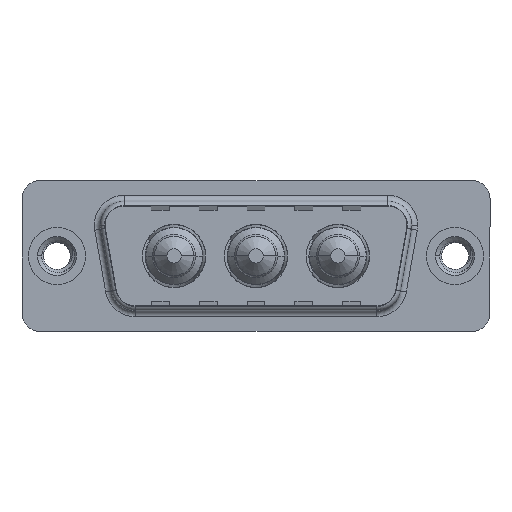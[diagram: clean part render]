
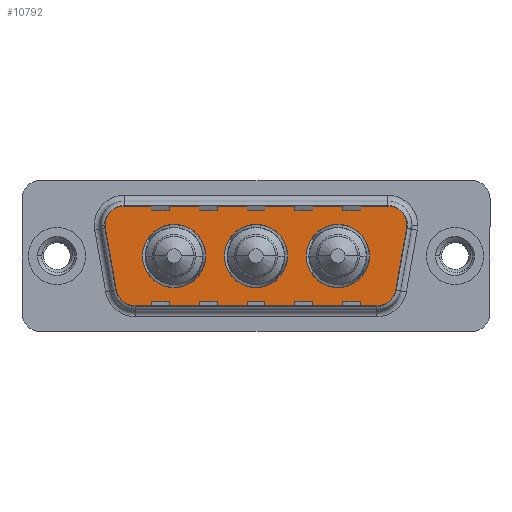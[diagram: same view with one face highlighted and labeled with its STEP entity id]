
A CAD part, top view. The second image highlights one B-rep face of the part: STEP entity #10792.
In plain terms, the highlighted planar face has unit normal (0, 0, 1).
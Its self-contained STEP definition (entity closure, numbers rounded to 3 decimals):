
#21 = LINE ( 'NONE', #7741, #7757 ) ;
#210 = CIRCLE ( 'NONE', #9782, 2. ) ;
#257 = ORIENTED_EDGE ( 'NONE', *, *, #7845, .F. ) ;
#334 = CIRCLE ( 'NONE', #1871, 2.65 ) ;
#369 = CARTESIAN_POINT ( 'NONE',  ( 12.45, 0., 0. ) ) ;
#437 = EDGE_CURVE ( 'NONE', #9714, #862, #210, .T. ) ;
#532 = AXIS2_PLACEMENT_3D ( 'NONE', #3360, #12889, #3415 ) ;
#657 = CIRCLE ( 'NONE', #532, 2. ) ;
#700 = CARTESIAN_POINT ( 'NONE',  ( 3.441, 2.553, 0. ) ) ;
#862 = VERTEX_POINT ( 'NONE', #700 ) ;
#1106 = CARTESIAN_POINT ( 'NONE',  ( 5.411, 4.9, 0. ) ) ;
#1285 = AXIS2_PLACEMENT_3D ( 'NONE', #4723, #5276, #8515 ) ;
#1311 = EDGE_LOOP ( 'NONE', ( #10219, #2895, #8151, #12848, #7768, #3499, #10234, #4878, #11126 ) ) ;
#1380 = AXIS2_PLACEMENT_3D ( 'NONE', #9017, #12062, #6514 ) ;
#1426 = CARTESIAN_POINT ( 'NONE',  ( 19.3, 0., 0. ) ) ;
#1620 = ORIENTED_EDGE ( 'NONE', *, *, #2970, .F. ) ;
#1871 = AXIS2_PLACEMENT_3D ( 'NONE', #4957, #11233, #6398 ) ;
#1946 = VERTEX_POINT ( 'NONE', #1426 ) ;
#2048 = EDGE_CURVE ( 'NONE', #12811, #10323, #3457, .T. ) ;
#2060 = FACE_BOUND ( 'NONE', #3068, .T. ) ;
#2156 = CIRCLE ( 'NONE', #4770, 2.65 ) ;
#2168 = CIRCLE ( 'NONE', #5638, 2. ) ;
#2248 = VERTEX_POINT ( 'NONE', #10719 ) ;
#2353 = AXIS2_PLACEMENT_3D ( 'NONE', #5855, #3461, #4319 ) ;
#2361 = CIRCLE ( 'NONE', #1380, 2.65 ) ;
#2462 = EDGE_CURVE ( 'NONE', #2248, #9714, #21, .T. ) ;
#2519 = DIRECTION ( 'NONE',  ( 0., 0., 1. ) ) ;
#2620 = DIRECTION ( 'NONE',  ( 1., 0., 0. ) ) ;
#2625 = AXIS2_PLACEMENT_3D ( 'NONE', #8718, #2669, #9718 ) ;
#2669 = DIRECTION ( 'NONE',  ( 0., 0., 1. ) ) ;
#2750 = DIRECTION ( 'NONE',  ( 0., 0., 1. ) ) ;
#2851 = CARTESIAN_POINT ( 'NONE',  ( 9.8, 0., 0. ) ) ;
#2853 = CARTESIAN_POINT ( 'NONE',  ( 9.8, 0., 0. ) ) ;
#2868 = CARTESIAN_POINT ( 'NONE',  ( 26.15, 0., 0. ) ) ;
#2895 = ORIENTED_EDGE ( 'NONE', *, *, #9051, .T. ) ;
#2924 = EDGE_CURVE ( 'NONE', #8588, #9337, #657, .T. ) ;
#2970 = EDGE_CURVE ( 'NONE', #6392, #9972, #334, .T. ) ;
#3068 = EDGE_LOOP ( 'NONE', ( #257, #5891 ) ) ;
#3135 = EDGE_LOOP ( 'NONE', ( #5721, #4028 ) ) ;
#3281 = AXIS2_PLACEMENT_3D ( 'NONE', #8675, #4645, #11713 ) ;
#3302 = CARTESIAN_POINT ( 'NONE',  ( 29.889, 2.9, 0. ) ) ;
#3360 = CARTESIAN_POINT ( 'NONE',  ( 27.889, 2.9, 0. ) ) ;
#3415 = DIRECTION ( 'NONE',  ( -1., 0., 0. ) ) ;
#3457 = CIRCLE ( 'NONE', #1285, 2. ) ;
#3461 = DIRECTION ( 'NONE',  ( 0., 0., 1. ) ) ;
#3499 = ORIENTED_EDGE ( 'NONE', *, *, #437, .T. ) ;
#3550 = EDGE_CURVE ( 'NONE', #5512, #1946, #2361, .T. ) ;
#3627 = EDGE_CURVE ( 'NONE', #10323, #10269, #6790, .T. ) ;
#3899 = CARTESIAN_POINT ( 'NONE',  ( 26.866, -4.9, 0. ) ) ;
#4028 = ORIENTED_EDGE ( 'NONE', *, *, #3550, .F. ) ;
#4207 = CARTESIAN_POINT ( 'NONE',  ( 3.441, 2.553, 0. ) ) ;
#4319 = DIRECTION ( 'NONE',  ( -1., 0., 0. ) ) ;
#4598 = PLANE ( 'NONE',  #3281 ) ;
#4645 = DIRECTION ( 'NONE',  ( 0., 0., 1. ) ) ;
#4723 = CARTESIAN_POINT ( 'NONE',  ( 6.434, -2.9, 0. ) ) ;
#4770 = AXIS2_PLACEMENT_3D ( 'NONE', #2851, #2750, #2620 ) ;
#4808 = LINE ( 'NONE', #11862, #5139 ) ;
#4878 = ORIENTED_EDGE ( 'NONE', *, *, #2048, .T. ) ;
#4957 = CARTESIAN_POINT ( 'NONE',  ( 23.5, 0., 0. ) ) ;
#5010 = CARTESIAN_POINT ( 'NONE',  ( 6.434, -4.9, 0. ) ) ;
#5139 = VECTOR ( 'NONE', #12114, 1000. ) ;
#5276 = DIRECTION ( 'NONE',  ( 0., 0., 1. ) ) ;
#5297 = CIRCLE ( 'NONE', #2353, 2. ) ;
#5326 = VERTEX_POINT ( 'NONE', #12324 ) ;
#5494 = EDGE_CURVE ( 'NONE', #5326, #7194, #2156, .T. ) ;
#5512 = VERTEX_POINT ( 'NONE', #8453 ) ;
#5638 = AXIS2_PLACEMENT_3D ( 'NONE', #12612, #2519, #11662 ) ;
#5721 = ORIENTED_EDGE ( 'NONE', *, *, #10802, .F. ) ;
#5735 = ORIENTED_EDGE ( 'NONE', *, *, #8368, .F. ) ;
#5816 = CARTESIAN_POINT ( 'NONE',  ( 5.411, 2.9, 0. ) ) ;
#5855 = CARTESIAN_POINT ( 'NONE',  ( 27.889, 2.9, 0. ) ) ;
#5891 = ORIENTED_EDGE ( 'NONE', *, *, #5494, .F. ) ;
#6178 = DIRECTION ( 'NONE',  ( 1., 0., 0. ) ) ;
#6253 = AXIS2_PLACEMENT_3D ( 'NONE', #8916, #8878, #8843 ) ;
#6392 = VERTEX_POINT ( 'NONE', #2868 ) ;
#6398 = DIRECTION ( 'NONE',  ( 1., 0., 0. ) ) ;
#6441 = CIRCLE ( 'NONE', #8776, 2.65 ) ;
#6514 = DIRECTION ( 'NONE',  ( 1., 0., 0. ) ) ;
#6790 = LINE ( 'NONE', #10793, #11831 ) ;
#7107 = CIRCLE ( 'NONE', #2625, 2.65 ) ;
#7194 = VERTEX_POINT ( 'NONE', #369 ) ;
#7214 = DIRECTION ( 'NONE',  ( 0.174, -0.985, 0. ) ) ;
#7293 = VERTEX_POINT ( 'NONE', #9871 ) ;
#7452 = EDGE_CURVE ( 'NONE', #10269, #7293, #2168, .T. ) ;
#7590 = VECTOR ( 'NONE', #7214, 1000. ) ;
#7741 = CARTESIAN_POINT ( 'NONE',  ( 5.411, 4.9, 0. ) ) ;
#7757 = VECTOR ( 'NONE', #13078, 1000. ) ;
#7768 = ORIENTED_EDGE ( 'NONE', *, *, #2462, .T. ) ;
#7845 = EDGE_CURVE ( 'NONE', #7194, #5326, #6441, .T. ) ;
#7851 = DIRECTION ( 'NONE',  ( 1., 0., 0. ) ) ;
#7907 = LINE ( 'NONE', #4207, #7590 ) ;
#8151 = ORIENTED_EDGE ( 'NONE', *, *, #2924, .T. ) ;
#8368 = EDGE_CURVE ( 'NONE', #9972, #6392, #9727, .T. ) ;
#8453 = CARTESIAN_POINT ( 'NONE',  ( 14., 0., 0. ) ) ;
#8515 = DIRECTION ( 'NONE',  ( -1., 0., 0. ) ) ;
#8588 = VERTEX_POINT ( 'NONE', #10704 ) ;
#8675 = CARTESIAN_POINT ( 'NONE',  ( 26.866, -2.9, 0. ) ) ;
#8718 = CARTESIAN_POINT ( 'NONE',  ( 16.65, 0., 0. ) ) ;
#8776 = AXIS2_PLACEMENT_3D ( 'NONE', #2853, #10661, #7851 ) ;
#8797 = EDGE_CURVE ( 'NONE', #9337, #2248, #5297, .T. ) ;
#8843 = DIRECTION ( 'NONE',  ( 1., 0., 0. ) ) ;
#8878 = DIRECTION ( 'NONE',  ( 0., 0., 1. ) ) ;
#8916 = CARTESIAN_POINT ( 'NONE',  ( 23.5, 0., 0. ) ) ;
#9017 = CARTESIAN_POINT ( 'NONE',  ( 16.65, 0., 0. ) ) ;
#9051 = EDGE_CURVE ( 'NONE', #7293, #8588, #4808, .T. ) ;
#9337 = VERTEX_POINT ( 'NONE', #3302 ) ;
#9366 = DIRECTION ( 'NONE',  ( 0., 0., 1. ) ) ;
#9490 = DIRECTION ( 'NONE',  ( 1., 0., 0. ) ) ;
#9714 = VERTEX_POINT ( 'NONE', #1106 ) ;
#9718 = DIRECTION ( 'NONE',  ( 1., 0., 0. ) ) ;
#9727 = CIRCLE ( 'NONE', #6253, 2.65 ) ;
#9782 = AXIS2_PLACEMENT_3D ( 'NONE', #5816, #9366, #9490 ) ;
#9871 = CARTESIAN_POINT ( 'NONE',  ( 28.836, -3.247, 0. ) ) ;
#9972 = VERTEX_POINT ( 'NONE', #10330 ) ;
#10086 = FACE_BOUND ( 'NONE', #3135, .T. ) ;
#10219 = ORIENTED_EDGE ( 'NONE', *, *, #7452, .T. ) ;
#10234 = ORIENTED_EDGE ( 'NONE', *, *, #10470, .T. ) ;
#10269 = VERTEX_POINT ( 'NONE', #3899 ) ;
#10323 = VERTEX_POINT ( 'NONE', #5010 ) ;
#10330 = CARTESIAN_POINT ( 'NONE',  ( 20.85, 0., 0. ) ) ;
#10470 = EDGE_CURVE ( 'NONE', #862, #12811, #7907, .T. ) ;
#10661 = DIRECTION ( 'NONE',  ( 0., 0., 1. ) ) ;
#10704 = CARTESIAN_POINT ( 'NONE',  ( 29.859, 2.553, 0. ) ) ;
#10719 = CARTESIAN_POINT ( 'NONE',  ( 27.889, 4.9, 0. ) ) ;
#10741 = CARTESIAN_POINT ( 'NONE',  ( 4.464, -3.247, 0. ) ) ;
#10792 = ADVANCED_FACE ( 'NONE', ( #10086, #12459, #2060, #12787 ), #4598, .T. ) ;
#10793 = CARTESIAN_POINT ( 'NONE',  ( 6.434, -4.9, 0. ) ) ;
#10802 = EDGE_CURVE ( 'NONE', #1946, #5512, #7107, .T. ) ;
#11126 = ORIENTED_EDGE ( 'NONE', *, *, #3627, .T. ) ;
#11233 = DIRECTION ( 'NONE',  ( 0., 0., 1. ) ) ;
#11286 = EDGE_LOOP ( 'NONE', ( #1620, #5735 ) ) ;
#11662 = DIRECTION ( 'NONE',  ( 1., 0., 0. ) ) ;
#11713 = DIRECTION ( 'NONE',  ( 1., 0., 0. ) ) ;
#11831 = VECTOR ( 'NONE', #6178, 1000. ) ;
#11862 = CARTESIAN_POINT ( 'NONE',  ( 29.859, 2.553, 0. ) ) ;
#12062 = DIRECTION ( 'NONE',  ( 0., 0., 1. ) ) ;
#12114 = DIRECTION ( 'NONE',  ( 0.174, 0.985, 0. ) ) ;
#12324 = CARTESIAN_POINT ( 'NONE',  ( 7.15, 0., 0. ) ) ;
#12459 = FACE_BOUND ( 'NONE', #11286, .T. ) ;
#12612 = CARTESIAN_POINT ( 'NONE',  ( 26.866, -2.9, 0. ) ) ;
#12787 = FACE_OUTER_BOUND ( 'NONE', #1311, .T. ) ;
#12811 = VERTEX_POINT ( 'NONE', #10741 ) ;
#12848 = ORIENTED_EDGE ( 'NONE', *, *, #8797, .T. ) ;
#12889 = DIRECTION ( 'NONE',  ( 0., 0., 1. ) ) ;
#13078 = DIRECTION ( 'NONE',  ( -1., 0., 0. ) ) ;
